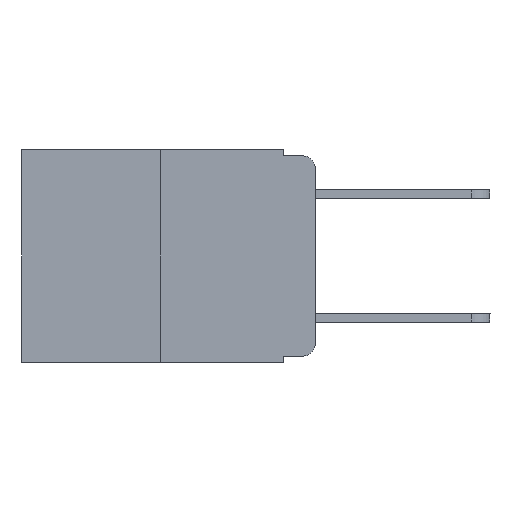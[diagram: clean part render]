
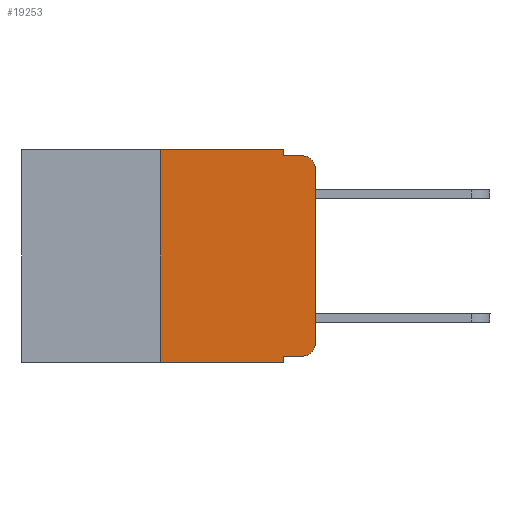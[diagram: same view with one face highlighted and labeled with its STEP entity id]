
A CAD part, left-side view. The second image highlights one B-rep face of the part: STEP entity #19253.
In plain terms, the highlighted planar face has unit normal (-1, 0, 0).
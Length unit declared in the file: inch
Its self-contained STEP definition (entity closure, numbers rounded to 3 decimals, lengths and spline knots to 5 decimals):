
#251 = VECTOR ( 'NONE', #3587, 39.37008 ) ;
#256 = ORIENTED_EDGE ( 'NONE', *, *, #18140, .T. ) ;
#263 = CARTESIAN_POINT ( 'NONE',  ( 0., 0.473, -0.343 ) ) ;
#730 = EDGE_CURVE ( 'NONE', #16777, #5246, #20665, .T. ) ;
#1081 = DIRECTION ( 'NONE',  ( 0., 0., -1. ) ) ;
#1888 = ORIENTED_EDGE ( 'NONE', *, *, #3982, .F. ) ;
#2380 = AXIS2_PLACEMENT_3D ( 'NONE', #3954, #3804, #9195 ) ;
#3012 = DIRECTION ( 'NONE',  ( -1., 0., 0. ) ) ;
#3074 = EDGE_CURVE ( 'NONE', #14279, #16148, #17830, .T. ) ;
#3507 = DIRECTION ( 'NONE',  ( 0., 0., -1. ) ) ;
#3587 = DIRECTION ( 'NONE',  ( 0., 0., 1. ) ) ;
#3708 = LINE ( 'NONE', #17412, #21629 ) ;
#3804 = DIRECTION ( 'NONE',  ( -1., 0., 0. ) ) ;
#3954 = CARTESIAN_POINT ( 'NONE',  ( 0., 0.02, -0.313 ) ) ;
#3970 = VERTEX_POINT ( 'NONE', #11479 ) ;
#3982 = EDGE_CURVE ( 'NONE', #9139, #16777, #3708, .T. ) ;
#4485 = ORIENTED_EDGE ( 'NONE', *, *, #10637, .F. ) ;
#4928 = EDGE_CURVE ( 'NONE', #12302, #14279, #21845, .T. ) ;
#5200 = DIRECTION ( 'NONE',  ( 0., 0., -1. ) ) ;
#5240 = PLANE ( 'NONE',  #21451 ) ;
#5246 = VERTEX_POINT ( 'NONE', #9109 ) ;
#6496 = CARTESIAN_POINT ( 'NONE',  ( 0., 0.051, -0.01 ) ) ;
#6728 = FACE_OUTER_BOUND ( 'NONE', #22221, .T. ) ;
#7035 = LINE ( 'NONE', #17386, #17029 ) ;
#7202 = CARTESIAN_POINT ( 'NONE',  ( 0., 0., 0. ) ) ;
#8087 = CARTESIAN_POINT ( 'NONE',  ( 0., 0.02, -0.03 ) ) ;
#8129 = AXIS2_PLACEMENT_3D ( 'NONE', #8087, #3012, #15071 ) ;
#8784 = EDGE_CURVE ( 'NONE', #18207, #13143, #7035, .T. ) ;
#8916 = EDGE_CURVE ( 'NONE', #16148, #5246, #18157, .T. ) ;
#9109 = CARTESIAN_POINT ( 'NONE',  ( 0., 0.02, -0.01 ) ) ;
#9139 = VERTEX_POINT ( 'NONE', #22095 ) ;
#9190 = ORIENTED_EDGE ( 'NONE', *, *, #3074, .T. ) ;
#9195 = DIRECTION ( 'NONE',  ( 0., 0., -1. ) ) ;
#9730 = CARTESIAN_POINT ( 'NONE',  ( 0., 0.25, 0. ) ) ;
#10579 = DIRECTION ( 'NONE',  ( 0., -1., 0. ) ) ;
#10637 = EDGE_CURVE ( 'NONE', #13143, #9139, #13325, .T. ) ;
#10819 = ORIENTED_EDGE ( 'NONE', *, *, #4928, .T. ) ;
#10822 = LINE ( 'NONE', #10889, #21417 ) ;
#10889 = CARTESIAN_POINT ( 'NONE',  ( 0., 0.051, -0.333 ) ) ;
#11479 = CARTESIAN_POINT ( 'NONE',  ( 0., 0.051, -0.333 ) ) ;
#12040 = CARTESIAN_POINT ( 'NONE',  ( 0., 0.473, 0. ) ) ;
#12171 = CARTESIAN_POINT ( 'NONE',  ( 0., 0., -0.03 ) ) ;
#12302 = VERTEX_POINT ( 'NONE', #14462 ) ;
#12634 = LINE ( 'NONE', #13055, #18365 ) ;
#13055 = CARTESIAN_POINT ( 'NONE',  ( 0., 0.051, 0. ) ) ;
#13143 = VERTEX_POINT ( 'NONE', #9730 ) ;
#13325 = LINE ( 'NONE', #15757, #18253 ) ;
#13548 = EDGE_CURVE ( 'NONE', #18207, #15725, #14010, .T. ) ;
#13767 = ORIENTED_EDGE ( 'NONE', *, *, #19722, .F. ) ;
#13826 = VECTOR ( 'NONE', #10579, 39.37008 ) ;
#14010 = LINE ( 'NONE', #263, #21924 ) ;
#14175 = CARTESIAN_POINT ( 'NONE',  ( 0., 0.25, -0.343 ) ) ;
#14279 = VERTEX_POINT ( 'NONE', #16847 ) ;
#14462 = CARTESIAN_POINT ( 'NONE',  ( 0., 0.02, -0.333 ) ) ;
#15071 = DIRECTION ( 'NONE',  ( 0., 0., -1. ) ) ;
#15473 = CARTESIAN_POINT ( 'NONE',  ( 0., 0.051, -0.01 ) ) ;
#15503 = DIRECTION ( 'NONE',  ( 1., 0., 0. ) ) ;
#15725 = VERTEX_POINT ( 'NONE', #21405 ) ;
#15757 = CARTESIAN_POINT ( 'NONE',  ( 0., 0.473, 0. ) ) ;
#16148 = VERTEX_POINT ( 'NONE', #12171 ) ;
#16151 = DIRECTION ( 'NONE',  ( 0., -1., 0. ) ) ;
#16488 = ORIENTED_EDGE ( 'NONE', *, *, #8784, .F. ) ;
#16777 = VERTEX_POINT ( 'NONE', #6496 ) ;
#16847 = CARTESIAN_POINT ( 'NONE',  ( 0., 0., -0.313 ) ) ;
#17029 = VECTOR ( 'NONE', #20722, 39.37008 ) ;
#17131 = DIRECTION ( 'NONE',  ( 0., -1., 0. ) ) ;
#17386 = CARTESIAN_POINT ( 'NONE',  ( 0., 0.25, 0. ) ) ;
#17412 = CARTESIAN_POINT ( 'NONE',  ( 0., 0.051, 0. ) ) ;
#17830 = LINE ( 'NONE', #7202, #251 ) ;
#17836 = ORIENTED_EDGE ( 'NONE', *, *, #13548, .T. ) ;
#18140 = EDGE_CURVE ( 'NONE', #3970, #12302, #10822, .T. ) ;
#18157 = CIRCLE ( 'NONE', #8129, 0.02 ) ;
#18207 = VERTEX_POINT ( 'NONE', #14175 ) ;
#18253 = VECTOR ( 'NONE', #17131, 39.37008 ) ;
#18365 = VECTOR ( 'NONE', #1081, 39.37008 ) ;
#19253 = ADVANCED_FACE ( 'NONE', ( #6728 ), #5240, .F. ) ;
#19415 = ORIENTED_EDGE ( 'NONE', *, *, #730, .F. ) ;
#19722 = EDGE_CURVE ( 'NONE', #3970, #15725, #12634, .T. ) ;
#20346 = ORIENTED_EDGE ( 'NONE', *, *, #8916, .T. ) ;
#20665 = LINE ( 'NONE', #15473, #13826 ) ;
#20722 = DIRECTION ( 'NONE',  ( 0., 0., 1. ) ) ;
#21179 = DIRECTION ( 'NONE',  ( 0., -1., 0. ) ) ;
#21405 = CARTESIAN_POINT ( 'NONE',  ( 0., 0.051, -0.343 ) ) ;
#21417 = VECTOR ( 'NONE', #16151, 39.37008 ) ;
#21451 = AXIS2_PLACEMENT_3D ( 'NONE', #12040, #15503, #3507 ) ;
#21629 = VECTOR ( 'NONE', #5200, 39.37008 ) ;
#21845 = CIRCLE ( 'NONE', #2380, 0.02 ) ;
#21924 = VECTOR ( 'NONE', #21179, 39.37008 ) ;
#22095 = CARTESIAN_POINT ( 'NONE',  ( 0., 0.051, 0. ) ) ;
#22221 = EDGE_LOOP ( 'NONE', ( #9190, #20346, #19415, #1888, #4485, #16488, #17836, #13767, #256, #10819 ) ) ;
